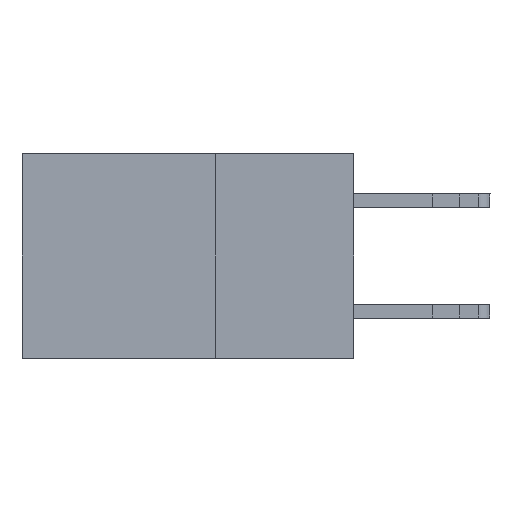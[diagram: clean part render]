
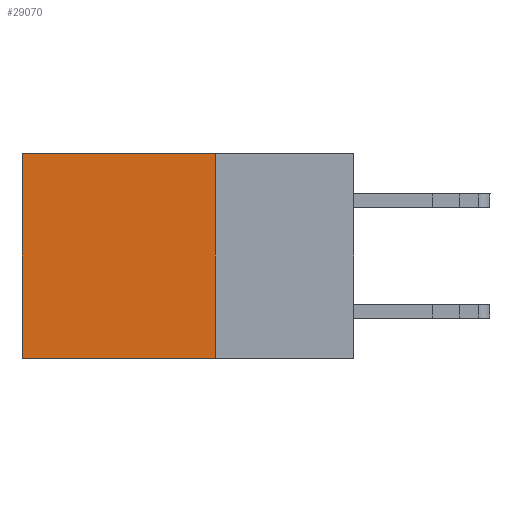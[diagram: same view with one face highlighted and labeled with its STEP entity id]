
A CAD part, left-side view. The second image highlights one B-rep face of the part: STEP entity #29070.
In plain terms, the highlighted planar face has unit normal (-1, 0, 0).
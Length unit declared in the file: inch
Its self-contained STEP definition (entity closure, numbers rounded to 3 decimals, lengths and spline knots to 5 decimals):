
#1246 = LINE ( 'NONE', #13118, #4888 ) ;
#1394 = VECTOR ( 'NONE', #28057, 39.37008 ) ;
#2235 = EDGE_CURVE ( 'NONE', #29167, #12110, #5436, .T. ) ;
#4451 = VECTOR ( 'NONE', #9346, 39.37008 ) ;
#4888 = VECTOR ( 'NONE', #21787, 39.37008 ) ;
#5436 = LINE ( 'NONE', #37183, #15322 ) ;
#9346 = DIRECTION ( 'NONE',  ( 0., 0., -1. ) ) ;
#10609 = VERTEX_POINT ( 'NONE', #15072 ) ;
#10631 = CARTESIAN_POINT ( 'NONE',  ( 0.2875, 0.6, 0. ) ) ;
#11062 = CARTESIAN_POINT ( 'NONE',  ( 0.2875, 0.6, -0.37 ) ) ;
#12110 = VERTEX_POINT ( 'NONE', #11062 ) ;
#12559 = EDGE_LOOP ( 'NONE', ( #12926, #21157, #12823, #13431 ) ) ;
#12567 = EDGE_CURVE ( 'NONE', #10609, #26079, #19406, .T. ) ;
#12823 = ORIENTED_EDGE ( 'NONE', *, *, #27673, .F. ) ;
#12926 = ORIENTED_EDGE ( 'NONE', *, *, #28537, .T. ) ;
#13118 = CARTESIAN_POINT ( 'NONE',  ( 0.2875, 0.6, 0. ) ) ;
#13431 = ORIENTED_EDGE ( 'NONE', *, *, #12567, .T. ) ;
#15072 = CARTESIAN_POINT ( 'NONE',  ( 0.2875, 0.25, 0. ) ) ;
#15322 = VECTOR ( 'NONE', #17005, 39.37008 ) ;
#17005 = DIRECTION ( 'NONE',  ( 0., 1., 0. ) ) ;
#19406 = LINE ( 'NONE', #36691, #1394 ) ;
#20725 = PLANE ( 'NONE',  #26239 ) ;
#21157 = ORIENTED_EDGE ( 'NONE', *, *, #2235, .F. ) ;
#21787 = DIRECTION ( 'NONE',  ( 0., 0., -1. ) ) ;
#22690 = CARTESIAN_POINT ( 'NONE',  ( 0.2875, 0.25, -0.37 ) ) ;
#23778 = LINE ( 'NONE', #29487, #4451 ) ;
#24176 = DIRECTION ( 'NONE',  ( 0., 0., -1. ) ) ;
#24308 = DIRECTION ( 'NONE',  ( 1., 0., 0. ) ) ;
#25971 = FACE_OUTER_BOUND ( 'NONE', #12559, .T. ) ;
#26079 = VERTEX_POINT ( 'NONE', #10631 ) ;
#26239 = AXIS2_PLACEMENT_3D ( 'NONE', #34843, #24308, #24176 ) ;
#27673 = EDGE_CURVE ( 'NONE', #10609, #29167, #23778, .T. ) ;
#28057 = DIRECTION ( 'NONE',  ( 0., 1., 0. ) ) ;
#28537 = EDGE_CURVE ( 'NONE', #26079, #12110, #1246, .T. ) ;
#29070 = ADVANCED_FACE ( 'NONE', ( #25971 ), #20725, .F. ) ;
#29167 = VERTEX_POINT ( 'NONE', #22690 ) ;
#29487 = CARTESIAN_POINT ( 'NONE',  ( 0.2875, 0.25, 0. ) ) ;
#34843 = CARTESIAN_POINT ( 'NONE',  ( 0.2875, 0.25, 0. ) ) ;
#36691 = CARTESIAN_POINT ( 'NONE',  ( 0.2875, 0.25, 0. ) ) ;
#37183 = CARTESIAN_POINT ( 'NONE',  ( 0.2875, 0.25, -0.37 ) ) ;
